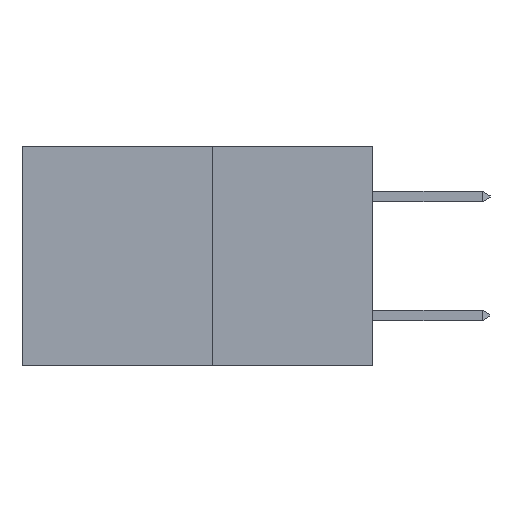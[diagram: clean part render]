
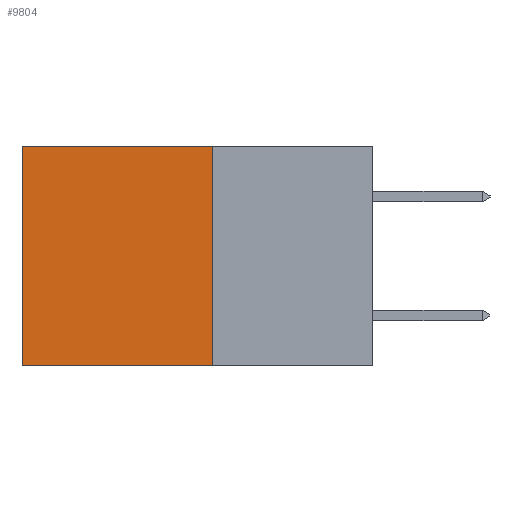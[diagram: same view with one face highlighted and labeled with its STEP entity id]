
A CAD part, left-side view. The second image highlights one B-rep face of the part: STEP entity #9804.
In plain terms, the highlighted planar face has unit normal (-1, 0, 0).
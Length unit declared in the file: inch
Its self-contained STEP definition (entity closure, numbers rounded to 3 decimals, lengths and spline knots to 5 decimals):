
#1026 = LINE ( 'NONE', #10940, #6958 ) ;
#1215 = PLANE ( 'NONE',  #6769 ) ;
#1571 = EDGE_CURVE ( 'NONE', #1740, #11432, #6045, .T. ) ;
#1587 = VERTEX_POINT ( 'NONE', #5685 ) ;
#1740 = VERTEX_POINT ( 'NONE', #13443 ) ;
#1754 = FACE_OUTER_BOUND ( 'NONE', #1911, .T. ) ;
#1779 = ORIENTED_EDGE ( 'NONE', *, *, #10247, .T. ) ;
#1911 = EDGE_LOOP ( 'NONE', ( #7634, #11496, #6990, #1779 ) ) ;
#1926 = DIRECTION ( 'NONE',  ( 0., 1., 0. ) ) ;
#2426 = DIRECTION ( 'NONE',  ( 1., 0., 0. ) ) ;
#2820 = DIRECTION ( 'NONE',  ( 0., 1., 0. ) ) ;
#2863 = DIRECTION ( 'NONE',  ( 0., 0., -1. ) ) ;
#4554 = LINE ( 'NONE', #8989, #7313 ) ;
#5685 = CARTESIAN_POINT ( 'NONE',  ( 0.277, 0.27, -0.37 ) ) ;
#6045 = LINE ( 'NONE', #11536, #12400 ) ;
#6578 = DIRECTION ( 'NONE',  ( 0., 0., -1. ) ) ;
#6769 = AXIS2_PLACEMENT_3D ( 'NONE', #9439, #2426, #10585 ) ;
#6958 = VECTOR ( 'NONE', #2863, 39.37008 ) ;
#6990 = ORIENTED_EDGE ( 'NONE', *, *, #11368, .F. ) ;
#7313 = VECTOR ( 'NONE', #1926, 39.37008 ) ;
#7491 = VECTOR ( 'NONE', #2820, 39.37008 ) ;
#7634 = ORIENTED_EDGE ( 'NONE', *, *, #1571, .T. ) ;
#8061 = VERTEX_POINT ( 'NONE', #13914 ) ;
#8234 = LINE ( 'NONE', #10947, #7491 ) ;
#8989 = CARTESIAN_POINT ( 'NONE',  ( 0.277, 0.27, 0. ) ) ;
#9439 = CARTESIAN_POINT ( 'NONE',  ( 0.277, 0.27, -0.37 ) ) ;
#9804 = ADVANCED_FACE ( 'NONE', ( #1754 ), #1215, .F. ) ;
#10247 = EDGE_CURVE ( 'NONE', #8061, #1740, #4554, .T. ) ;
#10585 = DIRECTION ( 'NONE',  ( 0., 0., -1. ) ) ;
#10940 = CARTESIAN_POINT ( 'NONE',  ( 0.277, 0.27, -0.37 ) ) ;
#10947 = CARTESIAN_POINT ( 'NONE',  ( 0.277, 0.27, -0.37 ) ) ;
#11368 = EDGE_CURVE ( 'NONE', #8061, #1587, #1026, .T. ) ;
#11432 = VERTEX_POINT ( 'NONE', #14189 ) ;
#11496 = ORIENTED_EDGE ( 'NONE', *, *, #12355, .F. ) ;
#11536 = CARTESIAN_POINT ( 'NONE',  ( 0.277, 0.59, -0.37 ) ) ;
#12355 = EDGE_CURVE ( 'NONE', #1587, #11432, #8234, .T. ) ;
#12400 = VECTOR ( 'NONE', #6578, 39.37008 ) ;
#13443 = CARTESIAN_POINT ( 'NONE',  ( 0.277, 0.59, 0. ) ) ;
#13914 = CARTESIAN_POINT ( 'NONE',  ( 0.277, 0.27, 0. ) ) ;
#14189 = CARTESIAN_POINT ( 'NONE',  ( 0.277, 0.59, -0.37 ) ) ;
